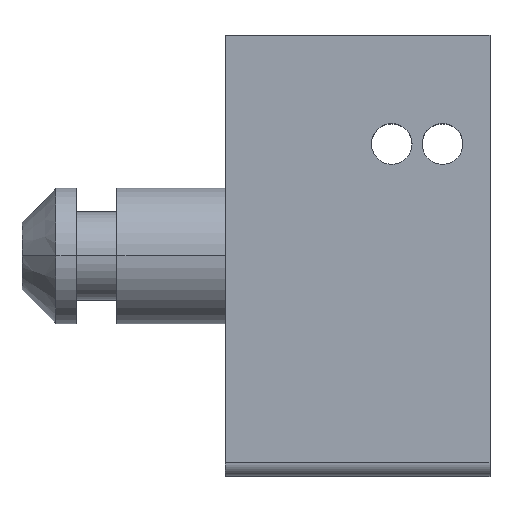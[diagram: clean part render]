
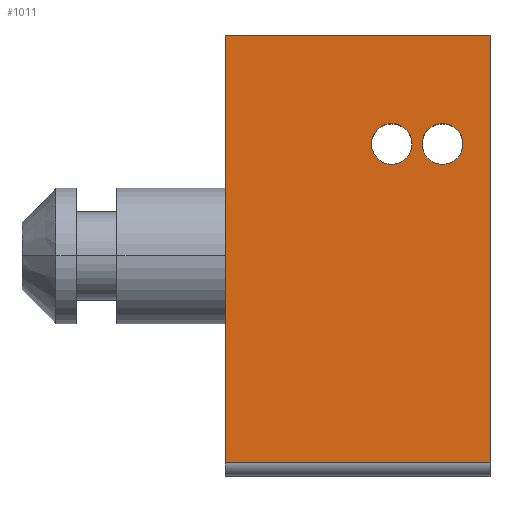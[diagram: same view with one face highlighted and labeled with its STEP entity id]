
A CAD part, top view. The second image highlights one B-rep face of the part: STEP entity #1011.
In plain terms, the highlighted planar face has unit normal (0, 0, 1).
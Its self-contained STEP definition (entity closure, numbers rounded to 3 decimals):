
#41 = DIRECTION ( 'NONE',  ( -1., 0., 0. ) ) ;
#67 = DIRECTION ( 'NONE',  ( 0., -1., 0. ) ) ;
#86 = CARTESIAN_POINT ( 'NONE',  ( 21., 49., 19. ) ) ;
#143 = EDGE_CURVE ( 'NONE', #602, #1226, #999, .T. ) ;
#162 = CARTESIAN_POINT ( 'NONE',  ( -11., 2., 19. ) ) ;
#202 = CIRCLE ( 'NONE', #338, 3. ) ;
#230 = CARTESIAN_POINT ( 'NONE',  ( 13.5, 49., 19. ) ) ;
#231 = VECTOR ( 'NONE', #713, 1000. ) ;
#235 = DIRECTION ( 'NONE',  ( 0., 0., 1. ) ) ;
#241 = VERTEX_POINT ( 'NONE', #386 ) ;
#244 = CARTESIAN_POINT ( 'NONE',  ( 10.5, 49., 19. ) ) ;
#248 = EDGE_CURVE ( 'NONE', #898, #1051, #291, .T. ) ;
#258 = DIRECTION ( 'NONE',  ( 0., 0., 1. ) ) ;
#266 = DIRECTION ( 'NONE',  ( -1., 0., 0. ) ) ;
#274 = EDGE_LOOP ( 'NONE', ( #691, #1030 ) ) ;
#277 = VERTEX_POINT ( 'NONE', #1085 ) ;
#291 = LINE ( 'NONE', #881, #1064 ) ;
#308 = CARTESIAN_POINT ( 'NONE',  ( 28., 2., 19. ) ) ;
#336 = DIRECTION ( 'NONE',  ( -1., 0., 0. ) ) ;
#338 = AXIS2_PLACEMENT_3D ( 'NONE', #1100, #594, #988 ) ;
#369 = ORIENTED_EDGE ( 'NONE', *, *, #823, .F. ) ;
#386 = CARTESIAN_POINT ( 'NONE',  ( 16.5, 49., 19. ) ) ;
#398 = EDGE_LOOP ( 'NONE', ( #838, #369 ) ) ;
#418 = AXIS2_PLACEMENT_3D ( 'NONE', #806, #608, #336 ) ;
#419 = EDGE_LOOP ( 'NONE', ( #882, #1145, #886, #710 ) ) ;
#421 = VECTOR ( 'NONE', #562, 1000. ) ;
#432 = FACE_BOUND ( 'NONE', #398, .T. ) ;
#444 = EDGE_CURVE ( 'NONE', #664, #277, #1220, .T. ) ;
#477 = AXIS2_PLACEMENT_3D ( 'NONE', #1114, #258, #524 ) ;
#478 = CARTESIAN_POINT ( 'NONE',  ( -11., 40., 19. ) ) ;
#520 = EDGE_CURVE ( 'NONE', #277, #664, #920, .T. ) ;
#524 = DIRECTION ( 'NONE',  ( -1., 0., 0. ) ) ;
#562 = DIRECTION ( 'NONE',  ( 0., -1., 0. ) ) ;
#594 = DIRECTION ( 'NONE',  ( 0., 0., 1. ) ) ;
#595 = AXIS2_PLACEMENT_3D ( 'NONE', #86, #742, #266 ) ;
#602 = VERTEX_POINT ( 'NONE', #162 ) ;
#608 = DIRECTION ( 'NONE',  ( 0., 0., -1. ) ) ;
#664 = VERTEX_POINT ( 'NONE', #932 ) ;
#691 = ORIENTED_EDGE ( 'NONE', *, *, #520, .F. ) ;
#695 = EDGE_CURVE ( 'NONE', #1051, #602, #1043, .T. ) ;
#710 = ORIENTED_EDGE ( 'NONE', *, *, #248, .T. ) ;
#713 = DIRECTION ( 'NONE',  ( 1., 0., 0. ) ) ;
#715 = DIRECTION ( 'NONE',  ( -1., 0., 0. ) ) ;
#736 = CARTESIAN_POINT ( 'NONE',  ( -11., 65., 19. ) ) ;
#742 = DIRECTION ( 'NONE',  ( 0., 0., 1. ) ) ;
#806 = CARTESIAN_POINT ( 'NONE',  ( -11., 40., 19. ) ) ;
#808 = CARTESIAN_POINT ( 'NONE',  ( -11., 2., 19. ) ) ;
#810 = EDGE_CURVE ( 'NONE', #898, #1226, #1187, .T. ) ;
#812 = PLANE ( 'NONE',  #418 ) ;
#820 = VERTEX_POINT ( 'NONE', #244 ) ;
#823 = EDGE_CURVE ( 'NONE', #241, #820, #202, .T. ) ;
#827 = EDGE_CURVE ( 'NONE', #820, #241, #1035, .T. ) ;
#838 = ORIENTED_EDGE ( 'NONE', *, *, #827, .F. ) ;
#881 = CARTESIAN_POINT ( 'NONE',  ( 0., 65., 19. ) ) ;
#882 = ORIENTED_EDGE ( 'NONE', *, *, #695, .T. ) ;
#886 = ORIENTED_EDGE ( 'NONE', *, *, #810, .F. ) ;
#898 = VERTEX_POINT ( 'NONE', #1178 ) ;
#912 = AXIS2_PLACEMENT_3D ( 'NONE', #230, #235, #715 ) ;
#920 = CIRCLE ( 'NONE', #477, 3. ) ;
#932 = CARTESIAN_POINT ( 'NONE',  ( 24., 49., 19. ) ) ;
#986 = CARTESIAN_POINT ( 'NONE',  ( 28., 40., 19. ) ) ;
#988 = DIRECTION ( 'NONE',  ( -1., 0., 0. ) ) ;
#999 = LINE ( 'NONE', #808, #231 ) ;
#1004 = FACE_BOUND ( 'NONE', #274, .T. ) ;
#1011 = ADVANCED_FACE ( 'NONE', ( #1004, #432, #1195 ), #812, .F. ) ;
#1030 = ORIENTED_EDGE ( 'NONE', *, *, #444, .F. ) ;
#1035 = CIRCLE ( 'NONE', #912, 3. ) ;
#1043 = LINE ( 'NONE', #478, #421 ) ;
#1051 = VERTEX_POINT ( 'NONE', #736 ) ;
#1064 = VECTOR ( 'NONE', #41, 1000. ) ;
#1085 = CARTESIAN_POINT ( 'NONE',  ( 18., 49., 19. ) ) ;
#1100 = CARTESIAN_POINT ( 'NONE',  ( 13.5, 49., 19. ) ) ;
#1101 = VECTOR ( 'NONE', #67, 1000. ) ;
#1114 = CARTESIAN_POINT ( 'NONE',  ( 21., 49., 19. ) ) ;
#1145 = ORIENTED_EDGE ( 'NONE', *, *, #143, .T. ) ;
#1178 = CARTESIAN_POINT ( 'NONE',  ( 28., 65., 19. ) ) ;
#1187 = LINE ( 'NONE', #986, #1101 ) ;
#1195 = FACE_OUTER_BOUND ( 'NONE', #419, .T. ) ;
#1220 = CIRCLE ( 'NONE', #595, 3. ) ;
#1226 = VERTEX_POINT ( 'NONE', #308 ) ;
